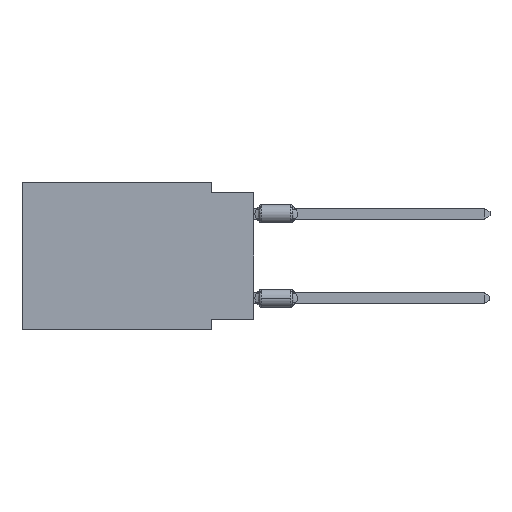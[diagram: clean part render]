
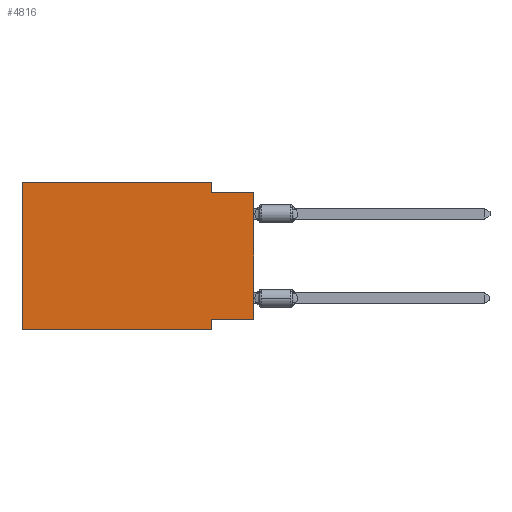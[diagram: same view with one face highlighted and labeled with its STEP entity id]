
A CAD part, left-side view. The second image highlights one B-rep face of the part: STEP entity #4816.
In plain terms, the highlighted planar face has unit normal (-1, 0, 0).
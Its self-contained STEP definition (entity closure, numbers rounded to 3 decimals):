
#451 = ORIENTED_EDGE ( 'NONE', *, *, #19686, .F. ) ;
#1594 = VECTOR ( 'NONE', #12398, 1000. ) ;
#1652 = LINE ( 'NONE', #8493, #19386 ) ;
#1661 = LINE ( 'NONE', #11758, #20941 ) ;
#1674 = CARTESIAN_POINT ( 'NONE',  ( 0., 0., -8.255 ) ) ;
#1785 = LINE ( 'NONE', #5355, #5372 ) ;
#2295 = VERTEX_POINT ( 'NONE', #18811 ) ;
#2598 = VERTEX_POINT ( 'NONE', #14991 ) ;
#2632 = CARTESIAN_POINT ( 'NONE',  ( 0., 13.97, 0. ) ) ;
#2878 = DIRECTION ( 'NONE',  ( 0., 1., 0. ) ) ;
#2918 = CARTESIAN_POINT ( 'NONE',  ( 0., 13.97, 0. ) ) ;
#3107 = ORIENTED_EDGE ( 'NONE', *, *, #4274, .F. ) ;
#4217 = DIRECTION ( 'NONE',  ( 0., 0., -1. ) ) ;
#4274 = EDGE_CURVE ( 'NONE', #6457, #16124, #14141, .T. ) ;
#4336 = DIRECTION ( 'NONE',  ( 1., 0., 0. ) ) ;
#4557 = DIRECTION ( 'NONE',  ( 0., 0., -1. ) ) ;
#4735 = CARTESIAN_POINT ( 'NONE',  ( 0., 13.97, -8.89 ) ) ;
#4816 = ADVANCED_FACE ( 'NONE', ( #7595 ), #14330, .F. ) ;
#4857 = LINE ( 'NONE', #11483, #8184 ) ;
#5346 = EDGE_CURVE ( 'NONE', #15819, #21123, #1661, .T. ) ;
#5355 = CARTESIAN_POINT ( 'NONE',  ( 0., 2.54, 0. ) ) ;
#5372 = VECTOR ( 'NONE', #10143, 1000. ) ;
#5663 = CARTESIAN_POINT ( 'NONE',  ( 0., 2.54, -0.635 ) ) ;
#6457 = VERTEX_POINT ( 'NONE', #4735 ) ;
#6479 = DIRECTION ( 'NONE',  ( 0., -1., 0. ) ) ;
#6811 = ORIENTED_EDGE ( 'NONE', *, *, #5346, .T. ) ;
#7595 = FACE_OUTER_BOUND ( 'NONE', #20379, .T. ) ;
#8043 = ORIENTED_EDGE ( 'NONE', *, *, #17443, .T. ) ;
#8184 = VECTOR ( 'NONE', #6479, 1000. ) ;
#8493 = CARTESIAN_POINT ( 'NONE',  ( 0., 13.97, -8.89 ) ) ;
#8547 = EDGE_CURVE ( 'NONE', #18830, #21123, #18885, .T. ) ;
#8714 = DIRECTION ( 'NONE',  ( 0., 0., 1. ) ) ;
#10143 = DIRECTION ( 'NONE',  ( 0., 0., -1. ) ) ;
#10460 = EDGE_CURVE ( 'NONE', #2598, #18830, #1785, .T. ) ;
#11012 = CARTESIAN_POINT ( 'NONE',  ( 0., 0., -0.635 ) ) ;
#11091 = ORIENTED_EDGE ( 'NONE', *, *, #16457, .F. ) ;
#11483 = CARTESIAN_POINT ( 'NONE',  ( 0., 13.97, 0. ) ) ;
#11733 = VECTOR ( 'NONE', #12350, 1000. ) ;
#11758 = CARTESIAN_POINT ( 'NONE',  ( 0., 0., 0. ) ) ;
#12350 = DIRECTION ( 'NONE',  ( 0., -1., 0. ) ) ;
#12398 = DIRECTION ( 'NONE',  ( 0., 0., 1. ) ) ;
#12468 = LINE ( 'NONE', #19104, #15648 ) ;
#14093 = CARTESIAN_POINT ( 'NONE',  ( 0., 0., -0.635 ) ) ;
#14141 = LINE ( 'NONE', #20772, #1594 ) ;
#14143 = EDGE_CURVE ( 'NONE', #16124, #2598, #4857, .T. ) ;
#14328 = ORIENTED_EDGE ( 'NONE', *, *, #10460, .F. ) ;
#14330 = PLANE ( 'NONE',  #16542 ) ;
#14914 = DIRECTION ( 'NONE',  ( 0., -1., 0. ) ) ;
#14991 = CARTESIAN_POINT ( 'NONE',  ( 0., 2.54, 0. ) ) ;
#15071 = CARTESIAN_POINT ( 'NONE',  ( 0., 2.54, -8.255 ) ) ;
#15648 = VECTOR ( 'NONE', #4217, 1000. ) ;
#15743 = ORIENTED_EDGE ( 'NONE', *, *, #14143, .F. ) ;
#15819 = VERTEX_POINT ( 'NONE', #1674 ) ;
#16124 = VERTEX_POINT ( 'NONE', #2632 ) ;
#16457 = EDGE_CURVE ( 'NONE', #16696, #2295, #12468, .T. ) ;
#16542 = AXIS2_PLACEMENT_3D ( 'NONE', #2918, #4336, #4557 ) ;
#16696 = VERTEX_POINT ( 'NONE', #15071 ) ;
#17443 = EDGE_CURVE ( 'NONE', #6457, #2295, #1652, .T. ) ;
#18627 = VECTOR ( 'NONE', #2878, 1000. ) ;
#18811 = CARTESIAN_POINT ( 'NONE',  ( 0., 2.54, -8.89 ) ) ;
#18830 = VERTEX_POINT ( 'NONE', #5663 ) ;
#18885 = LINE ( 'NONE', #14093, #11733 ) ;
#19104 = CARTESIAN_POINT ( 'NONE',  ( 0., 2.54, -8.89 ) ) ;
#19386 = VECTOR ( 'NONE', #14914, 1000. ) ;
#19396 = LINE ( 'NONE', #19601, #18627 ) ;
#19601 = CARTESIAN_POINT ( 'NONE',  ( 0., 0., -8.255 ) ) ;
#19686 = EDGE_CURVE ( 'NONE', #15819, #16696, #19396, .T. ) ;
#19784 = ORIENTED_EDGE ( 'NONE', *, *, #8547, .F. ) ;
#20379 = EDGE_LOOP ( 'NONE', ( #6811, #19784, #14328, #15743, #3107, #8043, #11091, #451 ) ) ;
#20772 = CARTESIAN_POINT ( 'NONE',  ( 0., 13.97, 0. ) ) ;
#20941 = VECTOR ( 'NONE', #8714, 1000. ) ;
#21123 = VERTEX_POINT ( 'NONE', #11012 ) ;
